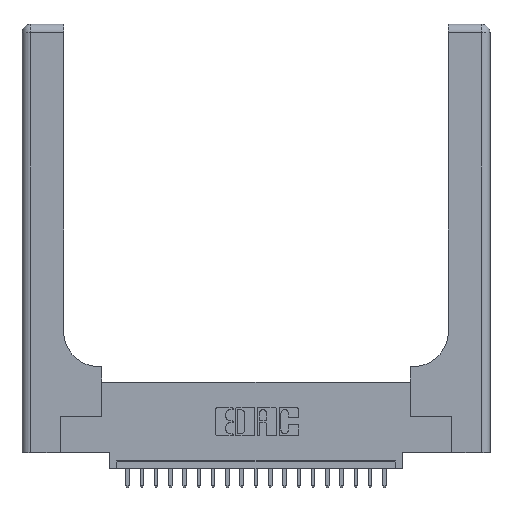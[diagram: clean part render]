
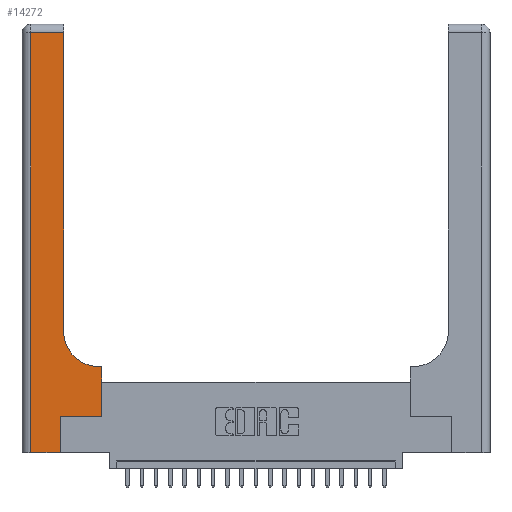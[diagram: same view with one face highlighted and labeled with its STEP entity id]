
A CAD part, top view. The second image highlights one B-rep face of the part: STEP entity #14272.
In plain terms, the highlighted planar face has unit normal (0, 0, 1).
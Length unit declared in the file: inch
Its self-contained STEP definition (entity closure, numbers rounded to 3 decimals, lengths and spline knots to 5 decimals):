
#236 = ORIENTED_EDGE ( 'NONE', *, *, #7207, .T. ) ;
#323 = DIRECTION ( 'NONE',  ( -1., 0., 0. ) ) ;
#347 = CARTESIAN_POINT ( 'NONE',  ( 0.2915, 3., 0.37 ) ) ;
#873 = DIRECTION ( 'NONE',  ( -1., 0., 0. ) ) ;
#1019 = CARTESIAN_POINT ( 'NONE',  ( 0., 2.94, 0.37 ) ) ;
#1152 = VERTEX_POINT ( 'NONE', #12642 ) ;
#1737 = CARTESIAN_POINT ( 'NONE',  ( 0.06, 2.94, 0.37 ) ) ;
#1960 = CIRCLE ( 'NONE', #17089, 0.25 ) ;
#2289 = DIRECTION ( 'NONE',  ( 1., 0., 0. ) ) ;
#2567 = CARTESIAN_POINT ( 'NONE',  ( 0.5415, 0.6, 0.37 ) ) ;
#3596 = EDGE_CURVE ( 'NONE', #8146, #7437, #9770, .T. ) ;
#3789 = CARTESIAN_POINT ( 'NONE',  ( 0.269, 0.25, 0.37 ) ) ;
#3815 = CARTESIAN_POINT ( 'NONE',  ( 0.269, 0.25, 0.37 ) ) ;
#3910 = CARTESIAN_POINT ( 'NONE',  ( 0.2915, 0.85, 0.37 ) ) ;
#3943 = EDGE_CURVE ( 'NONE', #12618, #1152, #10287, .T. ) ;
#3966 = CARTESIAN_POINT ( 'NONE',  ( 0., 0., 0.37 ) ) ;
#4480 = EDGE_CURVE ( 'NONE', #1152, #16340, #15746, .T. ) ;
#4715 = VERTEX_POINT ( 'NONE', #2567 ) ;
#5601 = VECTOR ( 'NONE', #9084, 39.37008 ) ;
#6290 = LINE ( 'NONE', #7179, #13711 ) ;
#6302 = CARTESIAN_POINT ( 'NONE',  ( 0.5415, 0.85, 0.37 ) ) ;
#6315 = VECTOR ( 'NONE', #7404, 39.37008 ) ;
#6404 = VECTOR ( 'NONE', #873, 39.37008 ) ;
#6526 = VECTOR ( 'NONE', #21272, 39.37008 ) ;
#7179 = CARTESIAN_POINT ( 'NONE',  ( 0.269, 0., 0.37 ) ) ;
#7207 = EDGE_CURVE ( 'NONE', #13224, #18067, #17840, .T. ) ;
#7223 = EDGE_CURVE ( 'NONE', #4715, #13224, #1960, .T. ) ;
#7404 = DIRECTION ( 'NONE',  ( 0., 1., 0. ) ) ;
#7437 = VERTEX_POINT ( 'NONE', #21175 ) ;
#7629 = ORIENTED_EDGE ( 'NONE', *, *, #13285, .T. ) ;
#8146 = VERTEX_POINT ( 'NONE', #17263 ) ;
#9084 = DIRECTION ( 'NONE',  ( 1., 0., 0. ) ) ;
#9770 = LINE ( 'NONE', #3966, #17706 ) ;
#10004 = CARTESIAN_POINT ( 'NONE',  ( 0.2915, 0.6, 0.37 ) ) ;
#10237 = ORIENTED_EDGE ( 'NONE', *, *, #18640, .T. ) ;
#10287 = LINE ( 'NONE', #3789, #5601 ) ;
#10368 = LINE ( 'NONE', #21504, #6526 ) ;
#10452 = ORIENTED_EDGE ( 'NONE', *, *, #7223, .T. ) ;
#10580 = DIRECTION ( 'NONE',  ( 0., 1., 0. ) ) ;
#10653 = ORIENTED_EDGE ( 'NONE', *, *, #4480, .T. ) ;
#11076 = LINE ( 'NONE', #1019, #6404 ) ;
#11415 = LINE ( 'NONE', #10004, #15498 ) ;
#12188 = AXIS2_PLACEMENT_3D ( 'NONE', #19415, #21211, #323 ) ;
#12618 = VERTEX_POINT ( 'NONE', #3815 ) ;
#12642 = CARTESIAN_POINT ( 'NONE',  ( 0.5585, 0.25, 0.37 ) ) ;
#13224 = VERTEX_POINT ( 'NONE', #3910 ) ;
#13285 = EDGE_CURVE ( 'NONE', #16340, #4715, #11415, .T. ) ;
#13481 = ORIENTED_EDGE ( 'NONE', *, *, #14846, .T. ) ;
#13711 = VECTOR ( 'NONE', #19290, 39.37008 ) ;
#14272 = ADVANCED_FACE ( 'NONE', ( #16009 ), #16046, .F. ) ;
#14846 = EDGE_CURVE ( 'NONE', #18067, #18590, #11076, .T. ) ;
#14907 = ORIENTED_EDGE ( 'NONE', *, *, #16835, .T. ) ;
#14928 = CARTESIAN_POINT ( 'NONE',  ( 0.5585, 0.25, 0.37 ) ) ;
#15498 = VECTOR ( 'NONE', #22297, 39.37008 ) ;
#15746 = LINE ( 'NONE', #14928, #22343 ) ;
#15850 = CARTESIAN_POINT ( 'NONE',  ( 0.5585, 0.6, 0.37 ) ) ;
#16009 = FACE_OUTER_BOUND ( 'NONE', #21035, .T. ) ;
#16046 = PLANE ( 'NONE',  #12188 ) ;
#16340 = VERTEX_POINT ( 'NONE', #15850 ) ;
#16726 = DIRECTION ( 'NONE',  ( 1., 0., 0. ) ) ;
#16835 = EDGE_CURVE ( 'NONE', #7437, #12618, #6290, .T. ) ;
#17089 = AXIS2_PLACEMENT_3D ( 'NONE', #6302, #18282, #16726 ) ;
#17263 = CARTESIAN_POINT ( 'NONE',  ( 0.06, 0., 0.37 ) ) ;
#17706 = VECTOR ( 'NONE', #2289, 39.37008 ) ;
#17840 = LINE ( 'NONE', #347, #6315 ) ;
#18067 = VERTEX_POINT ( 'NONE', #19388 ) ;
#18282 = DIRECTION ( 'NONE',  ( 0., 0., -1. ) ) ;
#18590 = VERTEX_POINT ( 'NONE', #1737 ) ;
#18640 = EDGE_CURVE ( 'NONE', #18590, #8146, #10368, .T. ) ;
#19290 = DIRECTION ( 'NONE',  ( 0., 1., 0. ) ) ;
#19388 = CARTESIAN_POINT ( 'NONE',  ( 0.2915, 2.94, 0.37 ) ) ;
#19415 = CARTESIAN_POINT ( 'NONE',  ( 0., 3., 0.37 ) ) ;
#20415 = ORIENTED_EDGE ( 'NONE', *, *, #3596, .T. ) ;
#21035 = EDGE_LOOP ( 'NONE', ( #236, #13481, #10237, #20415, #14907, #22091, #10653, #7629, #10452 ) ) ;
#21175 = CARTESIAN_POINT ( 'NONE',  ( 0.269, 0., 0.37 ) ) ;
#21211 = DIRECTION ( 'NONE',  ( 0., 0., -1. ) ) ;
#21272 = DIRECTION ( 'NONE',  ( 0., -1., 0. ) ) ;
#21504 = CARTESIAN_POINT ( 'NONE',  ( 0.06, 3., 0.37 ) ) ;
#22091 = ORIENTED_EDGE ( 'NONE', *, *, #3943, .T. ) ;
#22297 = DIRECTION ( 'NONE',  ( -1., 0., 0. ) ) ;
#22343 = VECTOR ( 'NONE', #10580, 39.37008 ) ;
